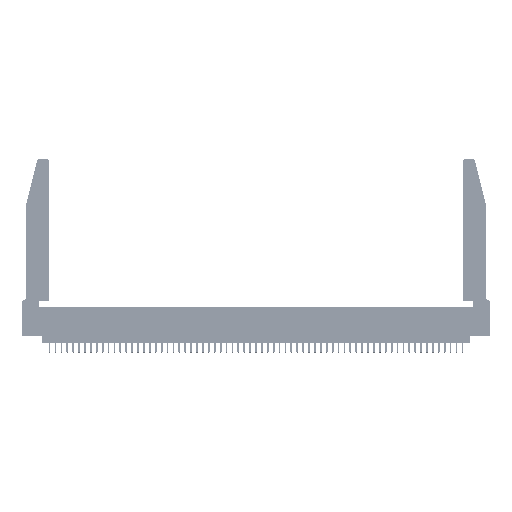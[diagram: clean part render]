
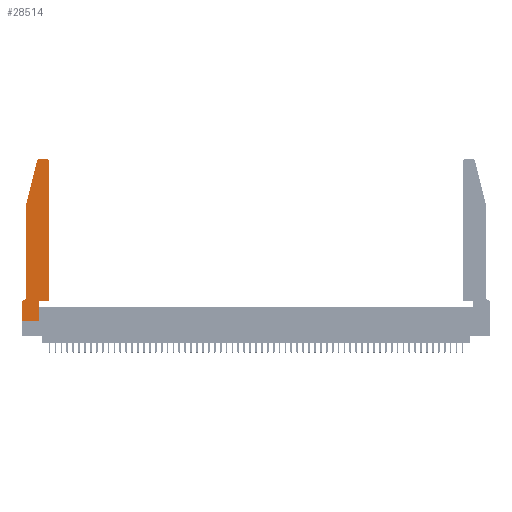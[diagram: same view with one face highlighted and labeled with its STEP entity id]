
A CAD part, top view. The second image highlights one B-rep face of the part: STEP entity #28514.
In plain terms, the highlighted planar face has unit normal (0, 0, 1).
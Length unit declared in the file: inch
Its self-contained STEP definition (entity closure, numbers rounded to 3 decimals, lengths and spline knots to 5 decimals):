
#477 = LINE ( 'NONE', #3132, #56088 ) ;
#866 = VERTEX_POINT ( 'NONE', #8894 ) ;
#1646 = LINE ( 'NONE', #54793, #23789 ) ;
#2081 = CIRCLE ( 'NONE', #11704, 0.03 ) ;
#2624 = ORIENTED_EDGE ( 'NONE', *, *, #56422, .T. ) ;
#3132 = CARTESIAN_POINT ( 'NONE',  ( 0.0755, 2., 0.37 ) ) ;
#3470 = EDGE_LOOP ( 'NONE', ( #9633, #24745, #32958, #32909, #2624, #36203, #54244, #4172, #39565, #5586, #9837, #11665 ) ) ;
#4172 = ORIENTED_EDGE ( 'NONE', *, *, #19068, .T. ) ;
#4300 = VERTEX_POINT ( 'NONE', #11606 ) ;
#5409 = CARTESIAN_POINT ( 'NONE',  ( 0., 0.35, 0.37 ) ) ;
#5469 = DIRECTION ( 'NONE',  ( 0., 1., 0. ) ) ;
#5586 = ORIENTED_EDGE ( 'NONE', *, *, #15023, .T. ) ;
#5883 = CIRCLE ( 'NONE', #51141, 0.07 ) ;
#6754 = VERTEX_POINT ( 'NONE', #49972 ) ;
#7246 = FACE_OUTER_BOUND ( 'NONE', #3470, .T. ) ;
#7424 = CARTESIAN_POINT ( 'NONE',  ( 0.0055, 0.42, 0.37 ) ) ;
#8422 = VERTEX_POINT ( 'NONE', #48677 ) ;
#8894 = CARTESIAN_POINT ( 'NONE',  ( 0., 0., 0.37 ) ) ;
#9633 = ORIENTED_EDGE ( 'NONE', *, *, #44643, .T. ) ;
#9837 = ORIENTED_EDGE ( 'NONE', *, *, #31977, .T. ) ;
#10244 = VECTOR ( 'NONE', #52664, 39.37008 ) ;
#10691 = EDGE_CURVE ( 'NONE', #4300, #29879, #33610, .T. ) ;
#11364 = VECTOR ( 'NONE', #25618, 39.37008 ) ;
#11587 = VECTOR ( 'NONE', #47207, 39.37008 ) ;
#11606 = CARTESIAN_POINT ( 'NONE',  ( 0.0055, 0.35, 0.37 ) ) ;
#11665 = ORIENTED_EDGE ( 'NONE', *, *, #33752, .T. ) ;
#11704 = AXIS2_PLACEMENT_3D ( 'NONE', #13452, #44036, #17836 ) ;
#11910 = DIRECTION ( 'NONE',  ( -1., 0., 0. ) ) ;
#12488 = CARTESIAN_POINT ( 'NONE',  ( 0.2865, 0.35, 0.37 ) ) ;
#13452 = CARTESIAN_POINT ( 'NONE',  ( 0.4205, 2.72, 0.37 ) ) ;
#14144 = CIRCLE ( 'NONE', #46517, 0.03 ) ;
#14335 = DIRECTION ( 'NONE',  ( 1., 0., 0. ) ) ;
#15023 = EDGE_CURVE ( 'NONE', #44322, #6754, #51607, .T. ) ;
#15110 = VERTEX_POINT ( 'NONE', #46603 ) ;
#15313 = DIRECTION ( 'NONE',  ( 0., -1., 0. ) ) ;
#15473 = CARTESIAN_POINT ( 'NONE',  ( 0., 0.35, 0.37 ) ) ;
#16202 = EDGE_CURVE ( 'NONE', #29879, #866, #39950, .T. ) ;
#17687 = CARTESIAN_POINT ( 'NONE',  ( 0.0755, 0.35, 0.37 ) ) ;
#17836 = DIRECTION ( 'NONE',  ( 1., 0., 0. ) ) ;
#18922 = LINE ( 'NONE', #32001, #52457 ) ;
#19068 = EDGE_CURVE ( 'NONE', #866, #51510, #23267, .T. ) ;
#20086 = EDGE_CURVE ( 'NONE', #51510, #44322, #52510, .T. ) ;
#21012 = CARTESIAN_POINT ( 'NONE',  ( 0., 0., 0.37 ) ) ;
#22150 = CARTESIAN_POINT ( 'NONE',  ( 0.284, 2.72, 0.37 ) ) ;
#23267 = LINE ( 'NONE', #21012, #11587 ) ;
#23789 = VECTOR ( 'NONE', #37440, 39.37008 ) ;
#24745 = ORIENTED_EDGE ( 'NONE', *, *, #54038, .T. ) ;
#25570 = AXIS2_PLACEMENT_3D ( 'NONE', #5409, #40532, #14335 ) ;
#25618 = DIRECTION ( 'NONE',  ( 0., 1., 0. ) ) ;
#26546 = DIRECTION ( 'NONE',  ( 1., 0., 0. ) ) ;
#27584 = DIRECTION ( 'NONE',  ( -1., 0., 0. ) ) ;
#28514 = ADVANCED_FACE ( 'NONE', ( #7246 ), #36176, .T. ) ;
#28691 = CARTESIAN_POINT ( 'NONE',  ( 0.0755, 2., 0.37 ) ) ;
#29378 = EDGE_CURVE ( 'NONE', #37974, #15110, #477, .T. ) ;
#29611 = CARTESIAN_POINT ( 'NONE',  ( 0.4505, 0.35, 0.37 ) ) ;
#29879 = VERTEX_POINT ( 'NONE', #15473 ) ;
#30765 = DIRECTION ( 'NONE',  ( 1., 0., 0. ) ) ;
#31133 = VECTOR ( 'NONE', #30765, 39.37008 ) ;
#31977 = EDGE_CURVE ( 'NONE', #6754, #55588, #36048, .T. ) ;
#32001 = CARTESIAN_POINT ( 'NONE',  ( 0.2605, 2.75, 0.37 ) ) ;
#32909 = ORIENTED_EDGE ( 'NONE', *, *, #29378, .T. ) ;
#32958 = ORIENTED_EDGE ( 'NONE', *, *, #53804, .T. ) ;
#33610 = LINE ( 'NONE', #17687, #10244 ) ;
#33752 = EDGE_CURVE ( 'NONE', #55588, #39563, #2081, .T. ) ;
#36048 = LINE ( 'NONE', #42963, #11364 ) ;
#36176 = PLANE ( 'NONE',  #25570 ) ;
#36203 = ORIENTED_EDGE ( 'NONE', *, *, #10691, .T. ) ;
#36739 = CARTESIAN_POINT ( 'NONE',  ( 0.25487, 2.72718, 0.37 ) ) ;
#36884 = CARTESIAN_POINT ( 'NONE',  ( 0.4505, 2.72, 0.37 ) ) ;
#37440 = DIRECTION ( 'NONE',  ( -0.239, -0.971, 0. ) ) ;
#37974 = VERTEX_POINT ( 'NONE', #28691 ) ;
#38122 = DIRECTION ( 'NONE',  ( 0., 0., -1. ) ) ;
#38299 = DIRECTION ( 'NONE',  ( 0., -1., 0. ) ) ;
#39563 = VERTEX_POINT ( 'NONE', #56436 ) ;
#39565 = ORIENTED_EDGE ( 'NONE', *, *, #20086, .T. ) ;
#39950 = LINE ( 'NONE', #50314, #50198 ) ;
#40012 = CARTESIAN_POINT ( 'NONE',  ( 0.2865, 0., 0.37 ) ) ;
#40532 = DIRECTION ( 'NONE',  ( 0., 0., 1. ) ) ;
#42277 = VECTOR ( 'NONE', #5469, 39.37008 ) ;
#42723 = VERTEX_POINT ( 'NONE', #36739 ) ;
#42963 = CARTESIAN_POINT ( 'NONE',  ( 0.4505, 0.35, 0.37 ) ) ;
#44036 = DIRECTION ( 'NONE',  ( 0., 0., 1. ) ) ;
#44322 = VERTEX_POINT ( 'NONE', #12488 ) ;
#44643 = EDGE_CURVE ( 'NONE', #39563, #8422, #18922, .T. ) ;
#46517 = AXIS2_PLACEMENT_3D ( 'NONE', #22150, #52685, #26546 ) ;
#46603 = CARTESIAN_POINT ( 'NONE',  ( 0.0755, 0.42, 0.37 ) ) ;
#47207 = DIRECTION ( 'NONE',  ( 1., 0., 0. ) ) ;
#48677 = CARTESIAN_POINT ( 'NONE',  ( 0.284, 2.75, 0.37 ) ) ;
#49388 = CARTESIAN_POINT ( 'NONE',  ( 0.2865, 0.35, 0.37 ) ) ;
#49972 = CARTESIAN_POINT ( 'NONE',  ( 0.4505, 0.35, 0.37 ) ) ;
#50198 = VECTOR ( 'NONE', #15313, 39.37008 ) ;
#50314 = CARTESIAN_POINT ( 'NONE',  ( 0., 0., 0.37 ) ) ;
#51141 = AXIS2_PLACEMENT_3D ( 'NONE', #7424, #38122, #11910 ) ;
#51510 = VERTEX_POINT ( 'NONE', #40012 ) ;
#51607 = LINE ( 'NONE', #29611, #31133 ) ;
#52457 = VECTOR ( 'NONE', #27584, 39.37008 ) ;
#52510 = LINE ( 'NONE', #49388, #42277 ) ;
#52664 = DIRECTION ( 'NONE',  ( -1., 0., 0. ) ) ;
#52685 = DIRECTION ( 'NONE',  ( 0., 0., 1. ) ) ;
#53804 = EDGE_CURVE ( 'NONE', #42723, #37974, #1646, .T. ) ;
#54038 = EDGE_CURVE ( 'NONE', #8422, #42723, #14144, .T. ) ;
#54244 = ORIENTED_EDGE ( 'NONE', *, *, #16202, .T. ) ;
#54793 = CARTESIAN_POINT ( 'NONE',  ( 0.0755, 2., 0.37 ) ) ;
#55588 = VERTEX_POINT ( 'NONE', #36884 ) ;
#56088 = VECTOR ( 'NONE', #38299, 39.37008 ) ;
#56422 = EDGE_CURVE ( 'NONE', #15110, #4300, #5883, .T. ) ;
#56436 = CARTESIAN_POINT ( 'NONE',  ( 0.4205, 2.75, 0.37 ) ) ;
